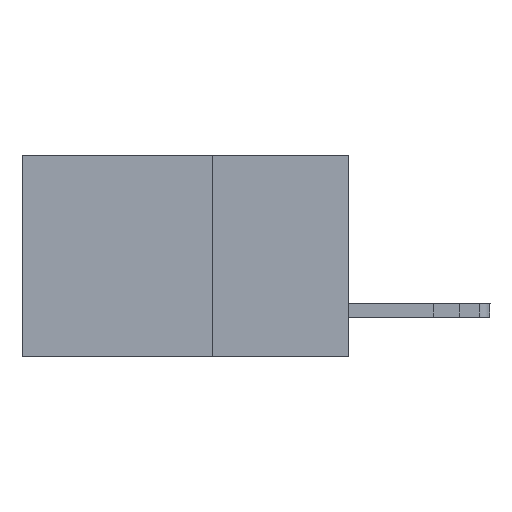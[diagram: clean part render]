
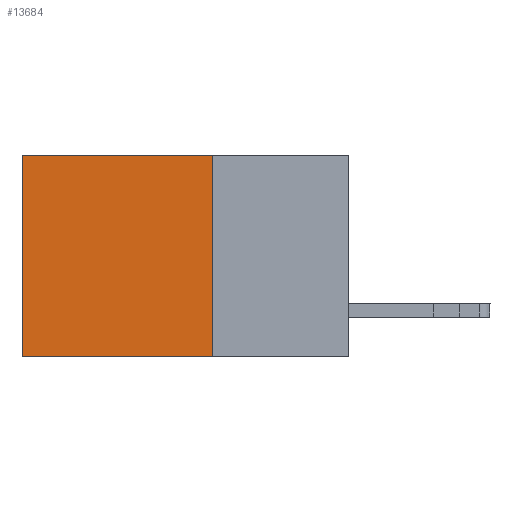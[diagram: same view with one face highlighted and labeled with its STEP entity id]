
A CAD part, left-side view. The second image highlights one B-rep face of the part: STEP entity #13684.
In plain terms, the highlighted planar face has unit normal (-1, 0, 0).
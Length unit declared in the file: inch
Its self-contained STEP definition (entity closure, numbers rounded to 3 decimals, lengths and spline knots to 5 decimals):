
#271 = DIRECTION ( 'NONE',  ( 0., 0., -1. ) ) ;
#668 = VECTOR ( 'NONE', #8859, 39.37008 ) ;
#1597 = PLANE ( 'NONE',  #12184 ) ;
#1760 = CARTESIAN_POINT ( 'NONE',  ( 0.298, 0.6, 0. ) ) ;
#2888 = VERTEX_POINT ( 'NONE', #6826 ) ;
#3968 = VERTEX_POINT ( 'NONE', #10875 ) ;
#4035 = CARTESIAN_POINT ( 'NONE',  ( 0.298, 0.25, 0. ) ) ;
#4234 = LINE ( 'NONE', #12553, #668 ) ;
#4611 = ORIENTED_EDGE ( 'NONE', *, *, #14604, .F. ) ;
#4828 = VECTOR ( 'NONE', #5572, 39.37008 ) ;
#5084 = EDGE_CURVE ( 'NONE', #2888, #12979, #10671, .T. ) ;
#5173 = VECTOR ( 'NONE', #7006, 39.37008 ) ;
#5211 = LINE ( 'NONE', #1760, #4828 ) ;
#5380 = LINE ( 'NONE', #15762, #5173 ) ;
#5572 = DIRECTION ( 'NONE',  ( 0., 0., -1. ) ) ;
#5586 = EDGE_LOOP ( 'NONE', ( #12887, #4611, #9938, #16227 ) ) ;
#6826 = CARTESIAN_POINT ( 'NONE',  ( 0.298, 0.25, 0. ) ) ;
#6851 = CARTESIAN_POINT ( 'NONE',  ( 0.298, 0.25, -0.37 ) ) ;
#7006 = DIRECTION ( 'NONE',  ( 0., 1., 0. ) ) ;
#7318 = VECTOR ( 'NONE', #14299, 39.37008 ) ;
#8473 = EDGE_CURVE ( 'NONE', #3968, #13567, #5211, .T. ) ;
#8859 = DIRECTION ( 'NONE',  ( 0., 1., 0. ) ) ;
#9293 = DIRECTION ( 'NONE',  ( 1., 0., 0. ) ) ;
#9355 = CARTESIAN_POINT ( 'NONE',  ( 0.298, 0.6, -0.37 ) ) ;
#9360 = FACE_OUTER_BOUND ( 'NONE', #5586, .T. ) ;
#9938 = ORIENTED_EDGE ( 'NONE', *, *, #5084, .F. ) ;
#10671 = LINE ( 'NONE', #13933, #7318 ) ;
#10875 = CARTESIAN_POINT ( 'NONE',  ( 0.298, 0.6, 0. ) ) ;
#12184 = AXIS2_PLACEMENT_3D ( 'NONE', #4035, #9293, #271 ) ;
#12553 = CARTESIAN_POINT ( 'NONE',  ( 0.298, 0.25, -0.37 ) ) ;
#12887 = ORIENTED_EDGE ( 'NONE', *, *, #8473, .T. ) ;
#12979 = VERTEX_POINT ( 'NONE', #6851 ) ;
#13567 = VERTEX_POINT ( 'NONE', #9355 ) ;
#13684 = ADVANCED_FACE ( 'NONE', ( #9360 ), #1597, .F. ) ;
#13933 = CARTESIAN_POINT ( 'NONE',  ( 0.298, 0.25, 0. ) ) ;
#14299 = DIRECTION ( 'NONE',  ( 0., 0., -1. ) ) ;
#14604 = EDGE_CURVE ( 'NONE', #12979, #13567, #4234, .T. ) ;
#15762 = CARTESIAN_POINT ( 'NONE',  ( 0.298, 0.25, 0. ) ) ;
#16227 = ORIENTED_EDGE ( 'NONE', *, *, #16313, .T. ) ;
#16313 = EDGE_CURVE ( 'NONE', #2888, #3968, #5380, .T. ) ;
